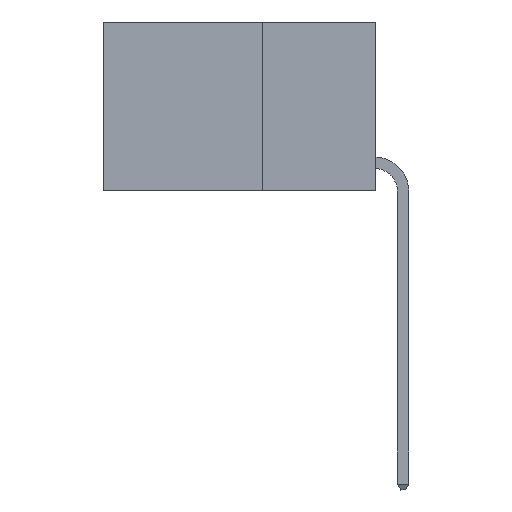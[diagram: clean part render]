
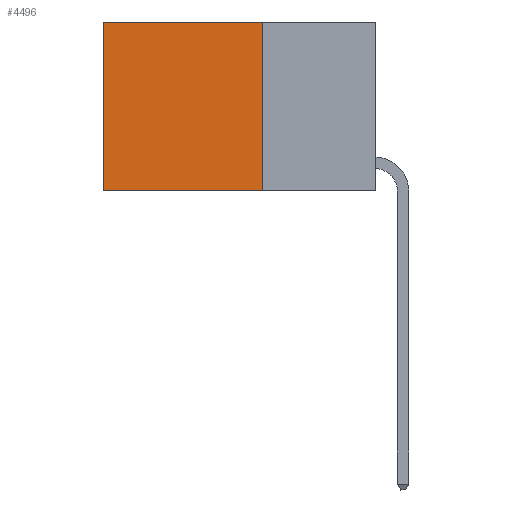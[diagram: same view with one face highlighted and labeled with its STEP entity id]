
A CAD part, left-side view. The second image highlights one B-rep face of the part: STEP entity #4496.
In plain terms, the highlighted planar face has unit normal (-1, 0, 0).
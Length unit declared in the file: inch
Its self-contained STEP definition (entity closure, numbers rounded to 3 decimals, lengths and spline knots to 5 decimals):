
#591 = VERTEX_POINT ( 'NONE', #8268 ) ;
#1169 = DIRECTION ( 'NONE',  ( 0., 0., -1. ) ) ;
#1245 = DIRECTION ( 'NONE',  ( 0., 0., -1. ) ) ;
#1308 = LINE ( 'NONE', #2437, #8549 ) ;
#1322 = CARTESIAN_POINT ( 'NONE',  ( 0.2625, 0.25, 0. ) ) ;
#1659 = DIRECTION ( 'NONE',  ( 0., 0., -1. ) ) ;
#1810 = ORIENTED_EDGE ( 'NONE', *, *, #11350, .T. ) ;
#1925 = LINE ( 'NONE', #8517, #8603 ) ;
#2275 = LINE ( 'NONE', #5730, #9214 ) ;
#2392 = CARTESIAN_POINT ( 'NONE',  ( 0.2625, 0.6, 0. ) ) ;
#2437 = CARTESIAN_POINT ( 'NONE',  ( 0.2625, 0.25, -0.37 ) ) ;
#2580 = VERTEX_POINT ( 'NONE', #2392 ) ;
#2688 = EDGE_LOOP ( 'NONE', ( #1810, #8719, #2824, #9583 ) ) ;
#2706 = CARTESIAN_POINT ( 'NONE',  ( 0.2625, 0.25, 0. ) ) ;
#2824 = ORIENTED_EDGE ( 'NONE', *, *, #8810, .F. ) ;
#2868 = DIRECTION ( 'NONE',  ( 1., 0., 0. ) ) ;
#4496 = ADVANCED_FACE ( 'NONE', ( #5405 ), #9610, .F. ) ;
#4538 = EDGE_CURVE ( 'NONE', #11408, #2580, #6949, .T. ) ;
#5195 = DIRECTION ( 'NONE',  ( 0., 1., 0. ) ) ;
#5405 = FACE_OUTER_BOUND ( 'NONE', #2688, .T. ) ;
#5730 = CARTESIAN_POINT ( 'NONE',  ( 0.2625, 0.25, 0. ) ) ;
#6708 = DIRECTION ( 'NONE',  ( 0., 1., 0. ) ) ;
#6887 = EDGE_CURVE ( 'NONE', #8937, #591, #1308, .T. ) ;
#6949 = LINE ( 'NONE', #7490, #9031 ) ;
#7490 = CARTESIAN_POINT ( 'NONE',  ( 0.2625, 0.25, 0. ) ) ;
#8268 = CARTESIAN_POINT ( 'NONE',  ( 0.2625, 0.6, -0.37 ) ) ;
#8517 = CARTESIAN_POINT ( 'NONE',  ( 0.2625, 0.6, 0. ) ) ;
#8549 = VECTOR ( 'NONE', #5195, 39.37008 ) ;
#8603 = VECTOR ( 'NONE', #1245, 39.37008 ) ;
#8719 = ORIENTED_EDGE ( 'NONE', *, *, #6887, .F. ) ;
#8810 = EDGE_CURVE ( 'NONE', #11408, #8937, #2275, .T. ) ;
#8937 = VERTEX_POINT ( 'NONE', #10304 ) ;
#9031 = VECTOR ( 'NONE', #6708, 39.37008 ) ;
#9214 = VECTOR ( 'NONE', #1169, 39.37008 ) ;
#9425 = AXIS2_PLACEMENT_3D ( 'NONE', #2706, #2868, #1659 ) ;
#9583 = ORIENTED_EDGE ( 'NONE', *, *, #4538, .T. ) ;
#9610 = PLANE ( 'NONE',  #9425 ) ;
#10304 = CARTESIAN_POINT ( 'NONE',  ( 0.2625, 0.25, -0.37 ) ) ;
#11350 = EDGE_CURVE ( 'NONE', #2580, #591, #1925, .T. ) ;
#11408 = VERTEX_POINT ( 'NONE', #1322 ) ;
